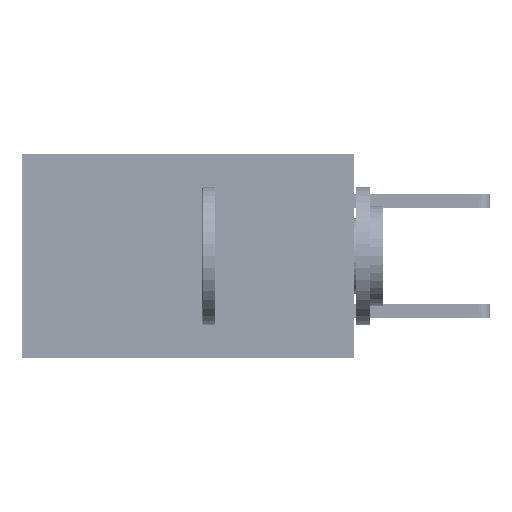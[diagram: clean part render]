
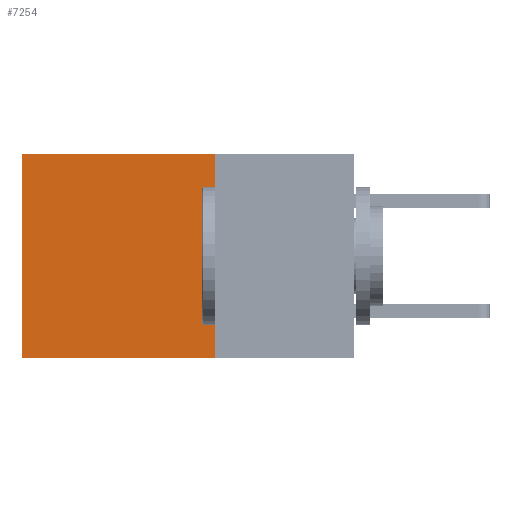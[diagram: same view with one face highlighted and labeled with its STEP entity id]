
A CAD part, left-side view. The second image highlights one B-rep face of the part: STEP entity #7254.
In plain terms, the highlighted planar face has unit normal (-1, 0, 0).
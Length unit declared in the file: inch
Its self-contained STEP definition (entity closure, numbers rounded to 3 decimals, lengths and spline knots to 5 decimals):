
#1897 = LINE ( 'NONE', #35345, #20432 ) ;
#3260 = CARTESIAN_POINT ( 'NONE',  ( 0.2875, 0.25, 0. ) ) ;
#4062 = CARTESIAN_POINT ( 'NONE',  ( 0.2875, 0.25, -0.37 ) ) ;
#4896 = DIRECTION ( 'NONE',  ( 0., 0., -1. ) ) ;
#5812 = ORIENTED_EDGE ( 'NONE', *, *, #21238, .T. ) ;
#6784 = CARTESIAN_POINT ( 'NONE',  ( 0.2875, 0.6, -0.37 ) ) ;
#7247 = ORIENTED_EDGE ( 'NONE', *, *, #16130, .F. ) ;
#7254 = ADVANCED_FACE ( 'NONE', ( #27307 ), #28006, .F. ) ;
#8860 = LINE ( 'NONE', #3260, #25852 ) ;
#13753 = CARTESIAN_POINT ( 'NONE',  ( 0.2875, 0.25, 0. ) ) ;
#15783 = LINE ( 'NONE', #25041, #34951 ) ;
#16130 = EDGE_CURVE ( 'NONE', #33028, #19562, #15783, .T. ) ;
#17835 = DIRECTION ( 'NONE',  ( 0., 1., 0. ) ) ;
#18345 = AXIS2_PLACEMENT_3D ( 'NONE', #13753, #24141, #27573 ) ;
#18641 = DIRECTION ( 'NONE',  ( 0., 0., -1. ) ) ;
#18896 = VERTEX_POINT ( 'NONE', #34955 ) ;
#19562 = VERTEX_POINT ( 'NONE', #41726 ) ;
#20432 = VECTOR ( 'NONE', #4896, 39.37008 ) ;
#21238 = EDGE_CURVE ( 'NONE', #18896, #21640, #1897, .T. ) ;
#21640 = VERTEX_POINT ( 'NONE', #6784 ) ;
#22487 = EDGE_CURVE ( 'NONE', #19562, #21640, #37457, .T. ) ;
#23430 = DIRECTION ( 'NONE',  ( 0., 1., 0. ) ) ;
#23887 = ORIENTED_EDGE ( 'NONE', *, *, #43857, .T. ) ;
#24141 = DIRECTION ( 'NONE',  ( 1., 0., 0. ) ) ;
#25041 = CARTESIAN_POINT ( 'NONE',  ( 0.2875, 0.25, 0. ) ) ;
#25852 = VECTOR ( 'NONE', #23430, 39.37008 ) ;
#27307 = FACE_OUTER_BOUND ( 'NONE', #35043, .T. ) ;
#27573 = DIRECTION ( 'NONE',  ( 0., 0., -1. ) ) ;
#28006 = PLANE ( 'NONE',  #18345 ) ;
#31191 = ORIENTED_EDGE ( 'NONE', *, *, #22487, .F. ) ;
#33028 = VERTEX_POINT ( 'NONE', #36465 ) ;
#34951 = VECTOR ( 'NONE', #18641, 39.37008 ) ;
#34955 = CARTESIAN_POINT ( 'NONE',  ( 0.2875, 0.6, 0. ) ) ;
#35043 = EDGE_LOOP ( 'NONE', ( #5812, #31191, #7247, #23887 ) ) ;
#35345 = CARTESIAN_POINT ( 'NONE',  ( 0.2875, 0.6, 0. ) ) ;
#36465 = CARTESIAN_POINT ( 'NONE',  ( 0.2875, 0.25, 0. ) ) ;
#37457 = LINE ( 'NONE', #4062, #42723 ) ;
#41726 = CARTESIAN_POINT ( 'NONE',  ( 0.2875, 0.25, -0.37 ) ) ;
#42723 = VECTOR ( 'NONE', #17835, 39.37008 ) ;
#43857 = EDGE_CURVE ( 'NONE', #33028, #18896, #8860, .T. ) ;
